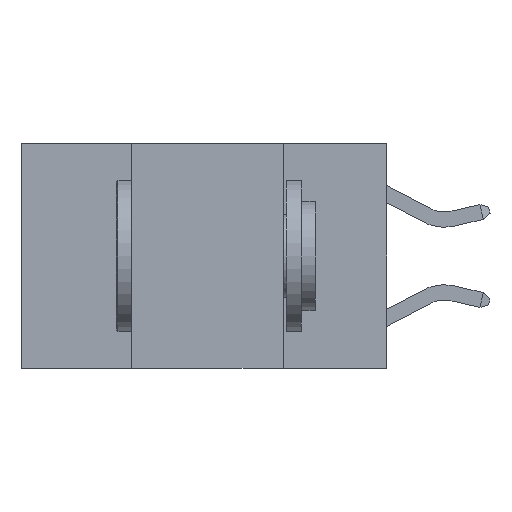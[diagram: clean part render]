
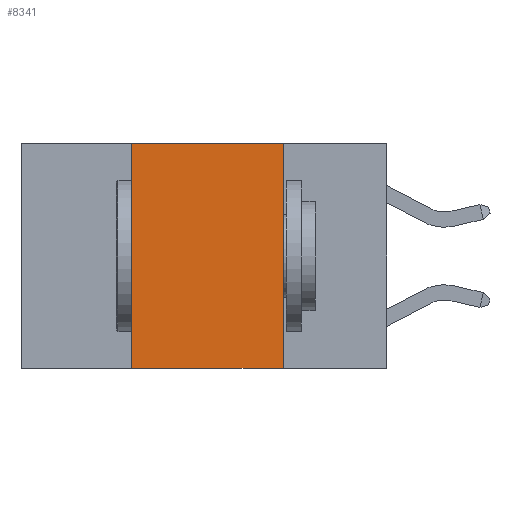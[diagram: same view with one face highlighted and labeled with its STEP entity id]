
A CAD part, left-side view. The second image highlights one B-rep face of the part: STEP entity #8341.
In plain terms, the highlighted planar face has unit normal (-1, 0, 0).
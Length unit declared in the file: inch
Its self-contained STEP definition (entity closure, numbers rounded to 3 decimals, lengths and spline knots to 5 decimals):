
#316 = PLANE ( 'NONE',  #6011 ) ;
#686 = LINE ( 'NONE', #1424, #15173 ) ;
#1126 = CARTESIAN_POINT ( 'NONE',  ( 0., 0.6, 0. ) ) ;
#1424 = CARTESIAN_POINT ( 'NONE',  ( 0., 0.17, 0. ) ) ;
#1749 = DIRECTION ( 'NONE',  ( 1., 0., 0. ) ) ;
#1820 = DIRECTION ( 'NONE',  ( 0., 0., 1. ) ) ;
#2117 = EDGE_LOOP ( 'NONE', ( #13010, #12591, #6451, #8444 ) ) ;
#2552 = FACE_OUTER_BOUND ( 'NONE', #2117, .T. ) ;
#2859 = DIRECTION ( 'NONE',  ( 0., 0., -1. ) ) ;
#4719 = EDGE_CURVE ( 'NONE', #6376, #11982, #686, .T. ) ;
#5584 = VECTOR ( 'NONE', #6069, 39.37008 ) ;
#6011 = AXIS2_PLACEMENT_3D ( 'NONE', #10221, #1749, #11604 ) ;
#6069 = DIRECTION ( 'NONE',  ( 0., -1., 0. ) ) ;
#6376 = VERTEX_POINT ( 'NONE', #6710 ) ;
#6407 = LINE ( 'NONE', #11672, #6853 ) ;
#6451 = ORIENTED_EDGE ( 'NONE', *, *, #15337, .F. ) ;
#6477 = VECTOR ( 'NONE', #15162, 39.37008 ) ;
#6710 = CARTESIAN_POINT ( 'NONE',  ( 0., 0.17, 0. ) ) ;
#6853 = VECTOR ( 'NONE', #1820, 39.37008 ) ;
#7908 = CARTESIAN_POINT ( 'NONE',  ( 0., 0.17, -0.37 ) ) ;
#8341 = ADVANCED_FACE ( 'NONE', ( #2552 ), #316, .F. ) ;
#8444 = ORIENTED_EDGE ( 'NONE', *, *, #10965, .T. ) ;
#9240 = VERTEX_POINT ( 'NONE', #13354 ) ;
#9650 = CARTESIAN_POINT ( 'NONE',  ( 0., 0.42, -0.37 ) ) ;
#10221 = CARTESIAN_POINT ( 'NONE',  ( 0., 0.6, 0. ) ) ;
#10635 = LINE ( 'NONE', #14413, #5584 ) ;
#10829 = VERTEX_POINT ( 'NONE', #9650 ) ;
#10965 = EDGE_CURVE ( 'NONE', #10829, #11982, #10635, .T. ) ;
#11604 = DIRECTION ( 'NONE',  ( 0., 0., -1. ) ) ;
#11672 = CARTESIAN_POINT ( 'NONE',  ( 0., 0.42, 0. ) ) ;
#11982 = VERTEX_POINT ( 'NONE', #7908 ) ;
#12591 = ORIENTED_EDGE ( 'NONE', *, *, #12756, .F. ) ;
#12756 = EDGE_CURVE ( 'NONE', #9240, #6376, #14340, .T. ) ;
#13010 = ORIENTED_EDGE ( 'NONE', *, *, #4719, .F. ) ;
#13354 = CARTESIAN_POINT ( 'NONE',  ( 0., 0.42, 0. ) ) ;
#14340 = LINE ( 'NONE', #1126, #6477 ) ;
#14413 = CARTESIAN_POINT ( 'NONE',  ( 0., 0.6, -0.37 ) ) ;
#15162 = DIRECTION ( 'NONE',  ( 0., -1., 0. ) ) ;
#15173 = VECTOR ( 'NONE', #2859, 39.37008 ) ;
#15337 = EDGE_CURVE ( 'NONE', #10829, #9240, #6407, .T. ) ;
